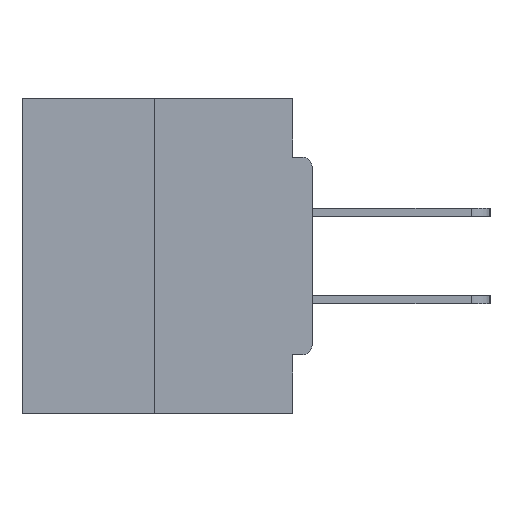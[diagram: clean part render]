
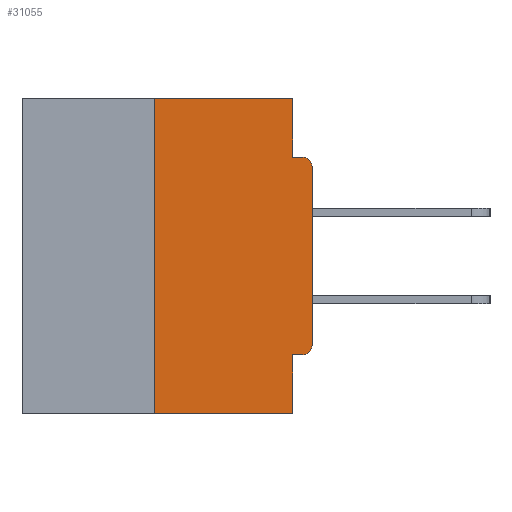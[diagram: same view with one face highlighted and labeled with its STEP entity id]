
A CAD part, left-side view. The second image highlights one B-rep face of the part: STEP entity #31055.
In plain terms, the highlighted planar face has unit normal (-1, 0, 0).
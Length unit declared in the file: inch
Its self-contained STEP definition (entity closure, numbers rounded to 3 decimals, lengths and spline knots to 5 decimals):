
#244 = CARTESIAN_POINT ( 'NONE',  ( 0., 0.25, 0. ) ) ;
#590 = CARTESIAN_POINT ( 'NONE',  ( 0., 0., 0. ) ) ;
#939 = VERTEX_POINT ( 'NONE', #8196 ) ;
#1271 = CARTESIAN_POINT ( 'NONE',  ( 0., 0.015, -0.3915 ) ) ;
#2046 = VECTOR ( 'NONE', #2124, 39.37008 ) ;
#2124 = DIRECTION ( 'NONE',  ( 0., -1., 0. ) ) ;
#2260 = EDGE_CURVE ( 'NONE', #22941, #14887, #4060, .T. ) ;
#2282 = DIRECTION ( 'NONE',  ( 0., 0., -1. ) ) ;
#2678 = VERTEX_POINT ( 'NONE', #10726 ) ;
#3177 = VERTEX_POINT ( 'NONE', #31191 ) ;
#3612 = EDGE_CURVE ( 'NONE', #19859, #3177, #17118, .T. ) ;
#3643 = DIRECTION ( 'NONE',  ( 0., -1., 0. ) ) ;
#3977 = VERTEX_POINT ( 'NONE', #22631 ) ;
#4060 = LINE ( 'NONE', #25998, #26845 ) ;
#4114 = FACE_OUTER_BOUND ( 'NONE', #22063, .T. ) ;
#4718 = DIRECTION ( 'NONE',  ( 1., 0., 0. ) ) ;
#4738 = VECTOR ( 'NONE', #5712, 39.37008 ) ;
#4845 = ORIENTED_EDGE ( 'NONE', *, *, #24210, .T. ) ;
#5712 = DIRECTION ( 'NONE',  ( 0., -1., 0. ) ) ;
#5964 = CARTESIAN_POINT ( 'NONE',  ( 0., 0., -0.4065 ) ) ;
#6180 = VERTEX_POINT ( 'NONE', #21475 ) ;
#6332 = VERTEX_POINT ( 'NONE', #8029 ) ;
#6738 = CARTESIAN_POINT ( 'NONE',  ( 0., 0.25, 0. ) ) ;
#7260 = CIRCLE ( 'NONE', #19402, 0.015 ) ;
#7339 = ORIENTED_EDGE ( 'NONE', *, *, #2260, .F. ) ;
#7641 = PLANE ( 'NONE',  #19883 ) ;
#7648 = EDGE_CURVE ( 'NONE', #6332, #22941, #28266, .T. ) ;
#7935 = EDGE_CURVE ( 'NONE', #3977, #3177, #14761, .T. ) ;
#8029 = CARTESIAN_POINT ( 'NONE',  ( 0., 0.25, -0.5 ) ) ;
#8196 = CARTESIAN_POINT ( 'NONE',  ( 0., 0.031, -0.5 ) ) ;
#8333 = CARTESIAN_POINT ( 'NONE',  ( 0., 0., -0.0935 ) ) ;
#8341 = DIRECTION ( 'NONE',  ( 0., 0., -1. ) ) ;
#8636 = DIRECTION ( 'NONE',  ( 0., 0., 1. ) ) ;
#9542 = EDGE_CURVE ( 'NONE', #2678, #6180, #20865, .T. ) ;
#10230 = ORIENTED_EDGE ( 'NONE', *, *, #24072, .F. ) ;
#10429 = CARTESIAN_POINT ( 'NONE',  ( 0., 0., -0.3915 ) ) ;
#10726 = CARTESIAN_POINT ( 'NONE',  ( 0., 0.015, -0.4065 ) ) ;
#10818 = DIRECTION ( 'NONE',  ( -1., 0., 0. ) ) ;
#11600 = DIRECTION ( 'NONE',  ( 0., 0., 1. ) ) ;
#11603 = CARTESIAN_POINT ( 'NONE',  ( 0., 0.015, -0.1085 ) ) ;
#12243 = DIRECTION ( 'NONE',  ( -1., 0., 0. ) ) ;
#12518 = CARTESIAN_POINT ( 'NONE',  ( 0., 0.46, 0. ) ) ;
#14728 = VECTOR ( 'NONE', #8636, 39.37008 ) ;
#14761 = CIRCLE ( 'NONE', #26184, 0.015 ) ;
#14887 = VERTEX_POINT ( 'NONE', #15161 ) ;
#15161 = CARTESIAN_POINT ( 'NONE',  ( 0., 0.031, 0. ) ) ;
#15275 = ORIENTED_EDGE ( 'NONE', *, *, #31657, .F. ) ;
#15677 = ORIENTED_EDGE ( 'NONE', *, *, #9542, .F. ) ;
#17118 = LINE ( 'NONE', #8333, #4738 ) ;
#17124 = CARTESIAN_POINT ( 'NONE',  ( 0., 0.031, -0.5 ) ) ;
#19038 = EDGE_CURVE ( 'NONE', #2678, #31721, #7260, .T. ) ;
#19402 = AXIS2_PLACEMENT_3D ( 'NONE', #1271, #10818, #8341 ) ;
#19859 = VERTEX_POINT ( 'NONE', #24995 ) ;
#19869 = CARTESIAN_POINT ( 'NONE',  ( 0., 0.46, -0.5 ) ) ;
#19883 = AXIS2_PLACEMENT_3D ( 'NONE', #12518, #4718, #21998 ) ;
#20667 = EDGE_CURVE ( 'NONE', #6332, #939, #30672, .T. ) ;
#20865 = LINE ( 'NONE', #5964, #21623 ) ;
#20995 = DIRECTION ( 'NONE',  ( 0., 1., 0. ) ) ;
#21475 = CARTESIAN_POINT ( 'NONE',  ( 0., 0.031, -0.4065 ) ) ;
#21623 = VECTOR ( 'NONE', #20995, 39.37008 ) ;
#21998 = DIRECTION ( 'NONE',  ( 0., 0., -1. ) ) ;
#22063 = EDGE_LOOP ( 'NONE', ( #7339, #27219, #30120, #15275, #15677, #22782, #4845, #31835, #29674, #10230 ) ) ;
#22631 = CARTESIAN_POINT ( 'NONE',  ( 0., 0., -0.1085 ) ) ;
#22782 = ORIENTED_EDGE ( 'NONE', *, *, #19038, .T. ) ;
#22941 = VERTEX_POINT ( 'NONE', #244 ) ;
#24072 = EDGE_CURVE ( 'NONE', #14887, #19859, #24725, .T. ) ;
#24150 = CARTESIAN_POINT ( 'NONE',  ( 0., 0.031, 0. ) ) ;
#24210 = EDGE_CURVE ( 'NONE', #31721, #3977, #27828, .T. ) ;
#24375 = DIRECTION ( 'NONE',  ( 0., 0., -1. ) ) ;
#24725 = LINE ( 'NONE', #24150, #26669 ) ;
#24995 = CARTESIAN_POINT ( 'NONE',  ( 0., 0.031, -0.0935 ) ) ;
#25946 = VECTOR ( 'NONE', #11600, 39.37008 ) ;
#25998 = CARTESIAN_POINT ( 'NONE',  ( 0., 0.46, 0. ) ) ;
#26184 = AXIS2_PLACEMENT_3D ( 'NONE', #11603, #12243, #29485 ) ;
#26491 = VECTOR ( 'NONE', #2282, 39.37008 ) ;
#26669 = VECTOR ( 'NONE', #24375, 39.37008 ) ;
#26845 = VECTOR ( 'NONE', #3643, 39.37008 ) ;
#27219 = ORIENTED_EDGE ( 'NONE', *, *, #7648, .F. ) ;
#27828 = LINE ( 'NONE', #590, #14728 ) ;
#28266 = LINE ( 'NONE', #6738, #25946 ) ;
#28430 = LINE ( 'NONE', #17124, #26491 ) ;
#29485 = DIRECTION ( 'NONE',  ( 0., 0., -1. ) ) ;
#29674 = ORIENTED_EDGE ( 'NONE', *, *, #3612, .F. ) ;
#30120 = ORIENTED_EDGE ( 'NONE', *, *, #20667, .T. ) ;
#30672 = LINE ( 'NONE', #19869, #2046 ) ;
#31055 = ADVANCED_FACE ( 'NONE', ( #4114 ), #7641, .F. ) ;
#31191 = CARTESIAN_POINT ( 'NONE',  ( 0., 0.015, -0.0935 ) ) ;
#31657 = EDGE_CURVE ( 'NONE', #6180, #939, #28430, .T. ) ;
#31721 = VERTEX_POINT ( 'NONE', #10429 ) ;
#31835 = ORIENTED_EDGE ( 'NONE', *, *, #7935, .T. ) ;
